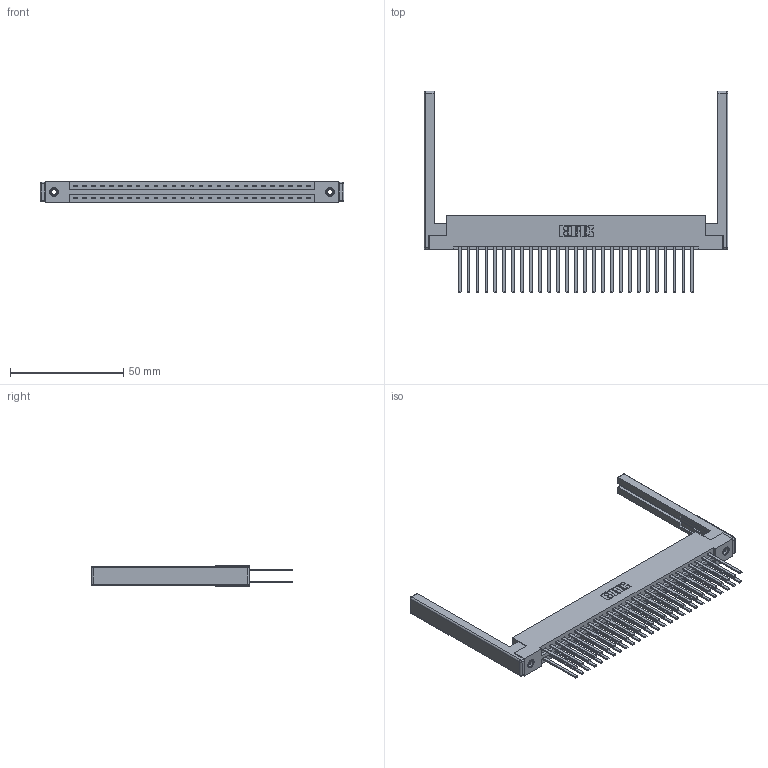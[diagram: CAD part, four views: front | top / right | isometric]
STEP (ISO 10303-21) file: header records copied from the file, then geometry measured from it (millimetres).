
FILE_DESCRIPTION (( 'STEP AP203' ), '1' );
FILE_NAME ('387-054-544-268.STEP', '2019-10-19T05:18:49', ( '' ), ( '' ), 'SwSTEP 2.0', 'SolidWorks 2016', '' );
FILE_SCHEMA (( 'CONFIG_CONTROL_DESIGN' ));
Length unit declared in the file: inch
Products named in the file (5): 387-054-544-268; 345-292-001_345-293-144; 345-250-001_345-250-001-102; 337 Part_Flush Mounting Lugs - 0.156 Dia-TI; 307-220-068
Assembly tree (59 placements, depth 2):
  387-054-544-268
    337 Part_Flush Mounting Lugs - 0.156 Dia-TI
    345-292-001_345-293-144  x54
    345-250-001_345-250-001-102  x2
    307-220-068  x2
Bounding box: 134.42 x 89.03 x 9.4 mm (x, y, z)
Volume: 19108 mm3; surface area: 23006.1 mm2
Topology: 59 solids, 59 shells, 2860 faces, 8423 edges, 5522 vertices
Faces by surface type: plane 1994, cylinder 842, cone 12, sphere 8, torus 4
Entity records: 25450 total; most frequent: CARTESIAN_POINT 4263, ORIENTED_EDGE 4188, DIRECTION 3720, EDGE_CURVE 2094, LINE 1920, VECTOR 1920, VERTEX_POINT 1386, AXIS2_PLACEMENT_3D 900
